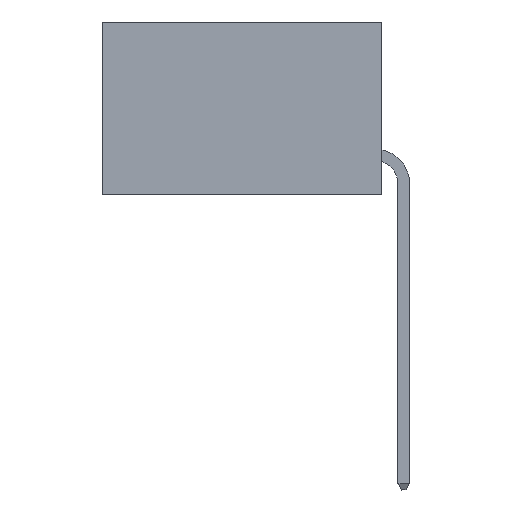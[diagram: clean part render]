
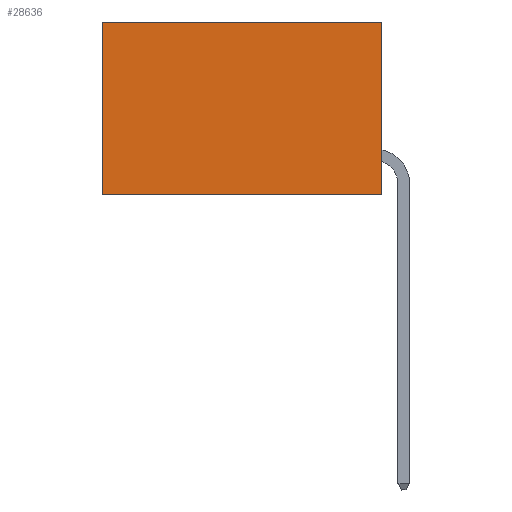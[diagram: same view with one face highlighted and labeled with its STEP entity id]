
A CAD part, left-side view. The second image highlights one B-rep face of the part: STEP entity #28636.
In plain terms, the highlighted planar face has unit normal (-1, 0, 0).
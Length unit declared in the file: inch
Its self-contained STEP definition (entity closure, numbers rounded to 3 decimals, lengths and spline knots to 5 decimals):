
#1583 = VERTEX_POINT ( 'NONE', #15919 ) ;
#2696 = CARTESIAN_POINT ( 'NONE',  ( 0.2875, 0., 0. ) ) ;
#4068 = EDGE_LOOP ( 'NONE', ( #11862, #24970, #44436, #16767 ) ) ;
#4996 = VECTOR ( 'NONE', #45850, 39.37008 ) ;
#5671 = EDGE_CURVE ( 'NONE', #28433, #1583, #14068, .T. ) ;
#6549 = PLANE ( 'NONE',  #17141 ) ;
#11862 = ORIENTED_EDGE ( 'NONE', *, *, #21915, .T. ) ;
#13545 = CARTESIAN_POINT ( 'NONE',  ( 0.2875, 0.6, 0. ) ) ;
#14068 = LINE ( 'NONE', #15865, #35868 ) ;
#15865 = CARTESIAN_POINT ( 'NONE',  ( 0.2875, 0., -0.37 ) ) ;
#15919 = CARTESIAN_POINT ( 'NONE',  ( 0.2875, 0.6, -0.37 ) ) ;
#16767 = ORIENTED_EDGE ( 'NONE', *, *, #18126, .T. ) ;
#17141 = AXIS2_PLACEMENT_3D ( 'NONE', #2696, #17743, #21607 ) ;
#17743 = DIRECTION ( 'NONE',  ( 1., 0., 0. ) ) ;
#18126 = EDGE_CURVE ( 'NONE', #36941, #38300, #39334, .T. ) ;
#20972 = EDGE_CURVE ( 'NONE', #36941, #28433, #40092, .T. ) ;
#21607 = DIRECTION ( 'NONE',  ( 0., 0., -1. ) ) ;
#21915 = EDGE_CURVE ( 'NONE', #38300, #1583, #46351, .T. ) ;
#22724 = CARTESIAN_POINT ( 'NONE',  ( 0.2875, 0., 0. ) ) ;
#24310 = DIRECTION ( 'NONE',  ( 0., 0., -1. ) ) ;
#24763 = CARTESIAN_POINT ( 'NONE',  ( 0.2875, 0.6, 0. ) ) ;
#24970 = ORIENTED_EDGE ( 'NONE', *, *, #5671, .F. ) ;
#28433 = VERTEX_POINT ( 'NONE', #43742 ) ;
#28636 = ADVANCED_FACE ( 'NONE', ( #46882 ), #6549, .F. ) ;
#33243 = CARTESIAN_POINT ( 'NONE',  ( 0.2875, 0., 0. ) ) ;
#35164 = CARTESIAN_POINT ( 'NONE',  ( 0.2875, 0., 0. ) ) ;
#35868 = VECTOR ( 'NONE', #45161, 39.37008 ) ;
#36941 = VERTEX_POINT ( 'NONE', #35164 ) ;
#37786 = DIRECTION ( 'NONE',  ( 0., 1., 0. ) ) ;
#38300 = VERTEX_POINT ( 'NONE', #24763 ) ;
#38743 = VECTOR ( 'NONE', #37786, 39.37008 ) ;
#39334 = LINE ( 'NONE', #22724, #38743 ) ;
#40092 = LINE ( 'NONE', #33243, #44051 ) ;
#43742 = CARTESIAN_POINT ( 'NONE',  ( 0.2875, 0., -0.37 ) ) ;
#44051 = VECTOR ( 'NONE', #24310, 39.37008 ) ;
#44436 = ORIENTED_EDGE ( 'NONE', *, *, #20972, .F. ) ;
#45161 = DIRECTION ( 'NONE',  ( 0., 1., 0. ) ) ;
#45850 = DIRECTION ( 'NONE',  ( 0., 0., -1. ) ) ;
#46351 = LINE ( 'NONE', #13545, #4996 ) ;
#46882 = FACE_OUTER_BOUND ( 'NONE', #4068, .T. ) ;
